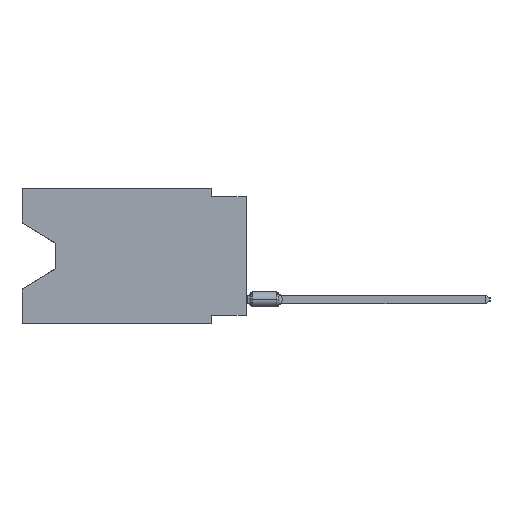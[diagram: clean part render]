
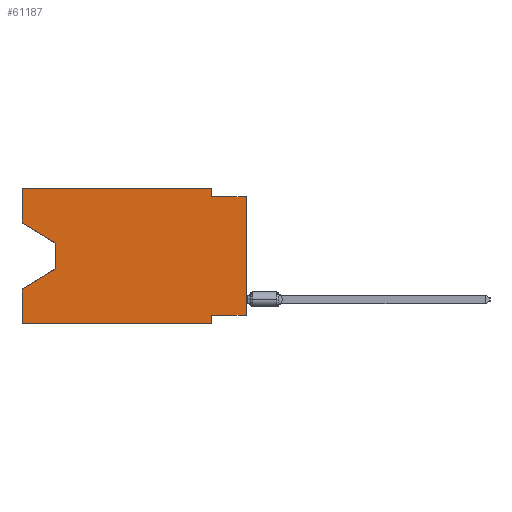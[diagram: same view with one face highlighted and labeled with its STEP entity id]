
A CAD part, left-side view. The second image highlights one B-rep face of the part: STEP entity #61187.
In plain terms, the highlighted planar face has unit normal (-1, 0, 0).
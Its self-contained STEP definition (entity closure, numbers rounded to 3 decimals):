
#321 = CARTESIAN_POINT ( 'NONE',  ( 0., 13.97, -5.893 ) ) ;
#675 = EDGE_CURVE ( 'NONE', #36463, #64387, #22153, .T. ) ;
#730 = LINE ( 'NONE', #20013, #17408 ) ;
#907 = EDGE_CURVE ( 'NONE', #5626, #34191, #730, .T. ) ;
#1509 = LINE ( 'NONE', #64002, #36518 ) ;
#1608 = CARTESIAN_POINT ( 'NONE',  ( 0., 2.54, -9.271 ) ) ;
#3417 = EDGE_CURVE ( 'NONE', #11963, #10879, #50940, .T. ) ;
#3717 = CARTESIAN_POINT ( 'NONE',  ( 0., 0., -0.635 ) ) ;
#3904 = CARTESIAN_POINT ( 'NONE',  ( 0., 2.54, 0. ) ) ;
#4790 = VECTOR ( 'NONE', #6890, 1000. ) ;
#5097 = VECTOR ( 'NONE', #7069, 1000. ) ;
#5626 = VERTEX_POINT ( 'NONE', #25548 ) ;
#6205 = LINE ( 'NONE', #17712, #55278 ) ;
#6890 = DIRECTION ( 'NONE',  ( 0., 0.855, -0.519 ) ) ;
#7069 = DIRECTION ( 'NONE',  ( 0., 1., 0. ) ) ;
#7502 = DIRECTION ( 'NONE',  ( 0., 0., -1. ) ) ;
#7621 = CARTESIAN_POINT ( 'NONE',  ( 0., 16.383, -9.906 ) ) ;
#8492 = PLANE ( 'NONE',  #21024 ) ;
#10879 = VERTEX_POINT ( 'NONE', #44319 ) ;
#11234 = VECTOR ( 'NONE', #45040, 1000. ) ;
#11963 = VERTEX_POINT ( 'NONE', #73167 ) ;
#12088 = ORIENTED_EDGE ( 'NONE', *, *, #47976, .T. ) ;
#12716 = VERTEX_POINT ( 'NONE', #19942 ) ;
#14358 = CARTESIAN_POINT ( 'NONE',  ( 0., 16.383, -2.546 ) ) ;
#15626 = LINE ( 'NONE', #3717, #59175 ) ;
#15627 = EDGE_CURVE ( 'NONE', #5626, #69040, #64213, .T. ) ;
#15860 = ORIENTED_EDGE ( 'NONE', *, *, #15627, .F. ) ;
#17408 = VECTOR ( 'NONE', #70181, 1000. ) ;
#17712 = CARTESIAN_POINT ( 'NONE',  ( 0., 2.54, 0. ) ) ;
#19665 = CARTESIAN_POINT ( 'NONE',  ( 0., 16.383, 0. ) ) ;
#19942 = CARTESIAN_POINT ( 'NONE',  ( 0., 2.54, -0.635 ) ) ;
#20013 = CARTESIAN_POINT ( 'NONE',  ( 0., 0., 0. ) ) ;
#20659 = CARTESIAN_POINT ( 'NONE',  ( 0., 16.383, 0. ) ) ;
#21024 = AXIS2_PLACEMENT_3D ( 'NONE', #77566, #45514, #70974 ) ;
#21697 = VERTEX_POINT ( 'NONE', #62709 ) ;
#22153 = LINE ( 'NONE', #14358, #29216 ) ;
#25548 = CARTESIAN_POINT ( 'NONE',  ( 0., 0., -9.271 ) ) ;
#26505 = LINE ( 'NONE', #7621, #11234 ) ;
#27193 = CARTESIAN_POINT ( 'NONE',  ( 0., 16.383, 0. ) ) ;
#28709 = EDGE_CURVE ( 'NONE', #69040, #21697, #1509, .T. ) ;
#29216 = VECTOR ( 'NONE', #72321, 1000. ) ;
#31908 = EDGE_CURVE ( 'NONE', #12716, #34191, #15626, .T. ) ;
#33141 = CARTESIAN_POINT ( 'NONE',  ( 0., 16.383, -2.546 ) ) ;
#33511 = VECTOR ( 'NONE', #44765, 1000. ) ;
#33790 = CARTESIAN_POINT ( 'NONE',  ( 0., 13.97, -5.893 ) ) ;
#33985 = FACE_OUTER_BOUND ( 'NONE', #79806, .T. ) ;
#34191 = VERTEX_POINT ( 'NONE', #35460 ) ;
#34593 = LINE ( 'NONE', #27193, #74466 ) ;
#34724 = VECTOR ( 'NONE', #53341, 1000. ) ;
#35460 = CARTESIAN_POINT ( 'NONE',  ( 0., 0., -0.635 ) ) ;
#36463 = VERTEX_POINT ( 'NONE', #33141 ) ;
#36518 = VECTOR ( 'NONE', #57835, 1000. ) ;
#36797 = ORIENTED_EDGE ( 'NONE', *, *, #31908, .F. ) ;
#39435 = ORIENTED_EDGE ( 'NONE', *, *, #50282, .T. ) ;
#42512 = VERTEX_POINT ( 'NONE', #20659 ) ;
#43137 = DIRECTION ( 'NONE',  ( 0., -1., 0. ) ) ;
#44319 = CARTESIAN_POINT ( 'NONE',  ( 0., 16.383, -7.36 ) ) ;
#44720 = LINE ( 'NONE', #321, #4790 ) ;
#44765 = DIRECTION ( 'NONE',  ( 0., 0., 1. ) ) ;
#44861 = ORIENTED_EDGE ( 'NONE', *, *, #78126, .T. ) ;
#45040 = DIRECTION ( 'NONE',  ( 0., -1., 0. ) ) ;
#45055 = ORIENTED_EDGE ( 'NONE', *, *, #3417, .F. ) ;
#45343 = CARTESIAN_POINT ( 'NONE',  ( 0., 13.97, -4.013 ) ) ;
#45514 = DIRECTION ( 'NONE',  ( 1., 0., 0. ) ) ;
#46213 = ORIENTED_EDGE ( 'NONE', *, *, #675, .T. ) ;
#46500 = VECTOR ( 'NONE', #7502, 1000. ) ;
#46512 = EDGE_CURVE ( 'NONE', #42512, #55911, #78812, .T. ) ;
#47976 = EDGE_CURVE ( 'NONE', #11963, #21697, #26505, .T. ) ;
#50282 = EDGE_CURVE ( 'NONE', #57249, #10879, #44720, .T. ) ;
#50940 = LINE ( 'NONE', #19665, #33511 ) ;
#53341 = DIRECTION ( 'NONE',  ( 0., -1., 0. ) ) ;
#54551 = CARTESIAN_POINT ( 'NONE',  ( 0., 16.383, 0. ) ) ;
#55278 = VECTOR ( 'NONE', #67891, 1000. ) ;
#55911 = VERTEX_POINT ( 'NONE', #3904 ) ;
#57170 = EDGE_CURVE ( 'NONE', #36463, #42512, #34593, .T. ) ;
#57249 = VERTEX_POINT ( 'NONE', #33790 ) ;
#57835 = DIRECTION ( 'NONE',  ( 0., 0., -1. ) ) ;
#59175 = VECTOR ( 'NONE', #43137, 1000. ) ;
#60152 = ORIENTED_EDGE ( 'NONE', *, *, #46512, .F. ) ;
#61187 = ADVANCED_FACE ( 'NONE', ( #33985 ), #8492, .F. ) ;
#62709 = CARTESIAN_POINT ( 'NONE',  ( 0., 2.54, -9.906 ) ) ;
#64002 = CARTESIAN_POINT ( 'NONE',  ( 0., 2.54, -9.906 ) ) ;
#64213 = LINE ( 'NONE', #75736, #5097 ) ;
#64387 = VERTEX_POINT ( 'NONE', #45343 ) ;
#64632 = DIRECTION ( 'NONE',  ( 0., 0., 1. ) ) ;
#65048 = CARTESIAN_POINT ( 'NONE',  ( 0., 13.97, -4.013 ) ) ;
#65579 = ORIENTED_EDGE ( 'NONE', *, *, #73594, .F. ) ;
#67891 = DIRECTION ( 'NONE',  ( 0., 0., -1. ) ) ;
#69040 = VERTEX_POINT ( 'NONE', #1608 ) ;
#70181 = DIRECTION ( 'NONE',  ( 0., 0., 1. ) ) ;
#70766 = ORIENTED_EDGE ( 'NONE', *, *, #28709, .F. ) ;
#70974 = DIRECTION ( 'NONE',  ( 0., 0., -1. ) ) ;
#72321 = DIRECTION ( 'NONE',  ( 0., -0.855, -0.519 ) ) ;
#73167 = CARTESIAN_POINT ( 'NONE',  ( 0., 16.383, -9.906 ) ) ;
#73594 = EDGE_CURVE ( 'NONE', #55911, #12716, #6205, .T. ) ;
#74466 = VECTOR ( 'NONE', #64632, 1000. ) ;
#75601 = ORIENTED_EDGE ( 'NONE', *, *, #907, .T. ) ;
#75736 = CARTESIAN_POINT ( 'NONE',  ( 0., 0., -9.271 ) ) ;
#76332 = ORIENTED_EDGE ( 'NONE', *, *, #57170, .F. ) ;
#77566 = CARTESIAN_POINT ( 'NONE',  ( 0., 16.383, 0. ) ) ;
#77782 = LINE ( 'NONE', #65048, #46500 ) ;
#78126 = EDGE_CURVE ( 'NONE', #64387, #57249, #77782, .T. ) ;
#78812 = LINE ( 'NONE', #54551, #34724 ) ;
#79806 = EDGE_LOOP ( 'NONE', ( #46213, #44861, #39435, #45055, #12088, #70766, #15860, #75601, #36797, #65579, #60152, #76332 ) ) ;
